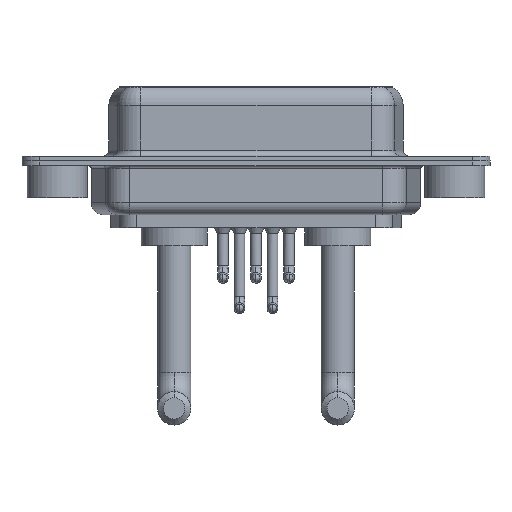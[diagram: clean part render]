
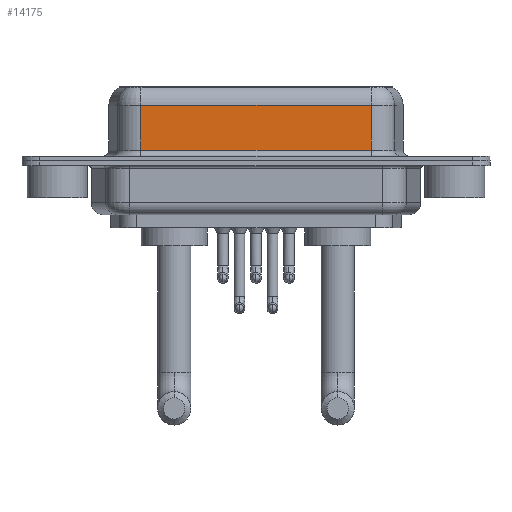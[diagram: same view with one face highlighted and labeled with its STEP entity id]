
A CAD part, front view. The second image highlights one B-rep face of the part: STEP entity #14175.
In plain terms, the highlighted planar face has unit normal (0, -1, 0).
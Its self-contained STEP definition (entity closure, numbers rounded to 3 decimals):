
#793 = CARTESIAN_POINT ( 'NONE',  ( 7.013, -3.95, 0.9 ) ) ;
#1282 = AXIS2_PLACEMENT_3D ( 'NONE', #11525, #2167, #8705 ) ;
#1319 = VERTEX_POINT ( 'NONE', #15889 ) ;
#1427 = EDGE_CURVE ( 'NONE', #11588, #1907, #5640, .T. ) ;
#1649 = CARTESIAN_POINT ( 'NONE',  ( 26.287, -3.95, 4.65 ) ) ;
#1703 = LINE ( 'NONE', #11923, #16756 ) ;
#1907 = VERTEX_POINT ( 'NONE', #5506 ) ;
#2167 = DIRECTION ( 'NONE',  ( 0., 1., 0. ) ) ;
#3400 = EDGE_CURVE ( 'NONE', #11588, #1319, #1703, .T. ) ;
#3539 = CARTESIAN_POINT ( 'NONE',  ( 7.013, -3.95, 6.4 ) ) ;
#4290 = DIRECTION ( 'NONE',  ( -1., 0., 0. ) ) ;
#4713 = FACE_OUTER_BOUND ( 'NONE', #15216, .T. ) ;
#5483 = CARTESIAN_POINT ( 'NONE',  ( 26.287, -3.95, 4.65 ) ) ;
#5506 = CARTESIAN_POINT ( 'NONE',  ( 7.013, -3.95, 4.65 ) ) ;
#5640 = LINE ( 'NONE', #1649, #14792 ) ;
#6030 = EDGE_CURVE ( 'NONE', #1907, #7866, #7351, .T. ) ;
#6090 = DIRECTION ( 'NONE',  ( 0., 0., -1. ) ) ;
#7047 = EDGE_CURVE ( 'NONE', #7866, #1319, #8434, .T. ) ;
#7351 = LINE ( 'NONE', #3539, #10495 ) ;
#7866 = VERTEX_POINT ( 'NONE', #793 ) ;
#7998 = ORIENTED_EDGE ( 'NONE', *, *, #7047, .T. ) ;
#8434 = LINE ( 'NONE', #8825, #15950 ) ;
#8705 = DIRECTION ( 'NONE',  ( 0., 0., 1. ) ) ;
#8825 = CARTESIAN_POINT ( 'NONE',  ( 26.287, -3.95, 0.9 ) ) ;
#9655 = ORIENTED_EDGE ( 'NONE', *, *, #3400, .F. ) ;
#10495 = VECTOR ( 'NONE', #6090, 1000. ) ;
#10819 = DIRECTION ( 'NONE',  ( 0., 0., -1. ) ) ;
#11466 = ORIENTED_EDGE ( 'NONE', *, *, #1427, .T. ) ;
#11525 = CARTESIAN_POINT ( 'NONE',  ( 26.287, -3.95, 6.4 ) ) ;
#11588 = VERTEX_POINT ( 'NONE', #5483 ) ;
#11923 = CARTESIAN_POINT ( 'NONE',  ( 26.287, -3.95, 6.4 ) ) ;
#13379 = ORIENTED_EDGE ( 'NONE', *, *, #6030, .T. ) ;
#13849 = PLANE ( 'NONE',  #1282 ) ;
#14175 = ADVANCED_FACE ( 'NONE', ( #4713 ), #13849, .F. ) ;
#14401 = DIRECTION ( 'NONE',  ( 1., 0., 0. ) ) ;
#14792 = VECTOR ( 'NONE', #4290, 1000. ) ;
#15216 = EDGE_LOOP ( 'NONE', ( #9655, #11466, #13379, #7998 ) ) ;
#15889 = CARTESIAN_POINT ( 'NONE',  ( 26.287, -3.95, 0.9 ) ) ;
#15950 = VECTOR ( 'NONE', #14401, 1000. ) ;
#16756 = VECTOR ( 'NONE', #10819, 1000. ) ;
